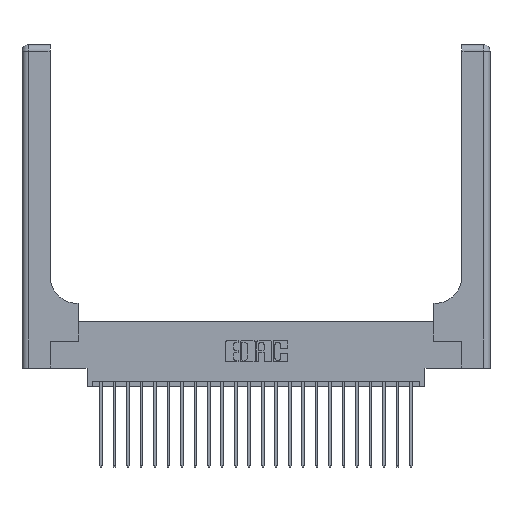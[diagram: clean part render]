
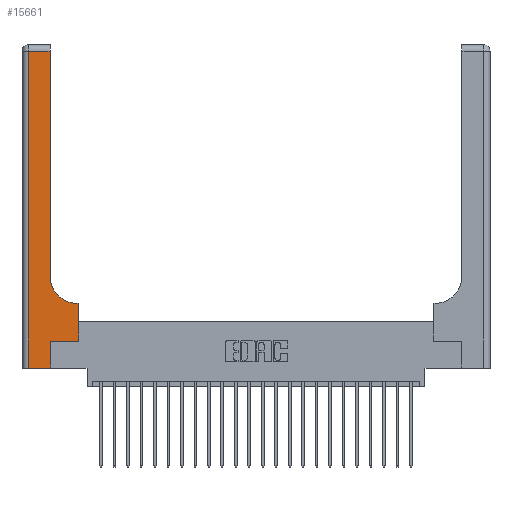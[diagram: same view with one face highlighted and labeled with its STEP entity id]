
A CAD part, top view. The second image highlights one B-rep face of the part: STEP entity #15661.
In plain terms, the highlighted planar face has unit normal (0, 0, 1).
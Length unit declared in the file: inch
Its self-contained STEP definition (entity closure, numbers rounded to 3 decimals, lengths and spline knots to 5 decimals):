
#237 = CARTESIAN_POINT ( 'NONE',  ( 0., 0., 0.37 ) ) ;
#488 = LINE ( 'NONE', #237, #18626 ) ;
#967 = EDGE_CURVE ( 'NONE', #19670, #8756, #488, .T. ) ;
#992 = CARTESIAN_POINT ( 'NONE',  ( 0.06, 2.94, 0.37 ) ) ;
#1204 = DIRECTION ( 'NONE',  ( 0., 1., 0. ) ) ;
#1926 = CARTESIAN_POINT ( 'NONE',  ( 0.26, 0.6, 0.37 ) ) ;
#2576 = FACE_OUTER_BOUND ( 'NONE', #18831, .T. ) ;
#2588 = ORIENTED_EDGE ( 'NONE', *, *, #967, .T. ) ;
#2594 = CARTESIAN_POINT ( 'NONE',  ( 0.528, 0.6, 0.37 ) ) ;
#3532 = VECTOR ( 'NONE', #5127, 39.37008 ) ;
#3684 = LINE ( 'NONE', #22855, #7391 ) ;
#3743 = CIRCLE ( 'NONE', #11062, 0.25 ) ;
#3860 = EDGE_CURVE ( 'NONE', #8756, #13955, #13489, .T. ) ;
#4247 = DIRECTION ( 'NONE',  ( 0., 1., 0. ) ) ;
#4313 = ORIENTED_EDGE ( 'NONE', *, *, #20091, .T. ) ;
#4708 = CARTESIAN_POINT ( 'NONE',  ( 0.51, 0.85, 0.37 ) ) ;
#4880 = ORIENTED_EDGE ( 'NONE', *, *, #19027, .T. ) ;
#5127 = DIRECTION ( 'NONE',  ( 0., -1., 0. ) ) ;
#5379 = EDGE_CURVE ( 'NONE', #11005, #16145, #3743, .T. ) ;
#5455 = ORIENTED_EDGE ( 'NONE', *, *, #5379, .T. ) ;
#5693 = CARTESIAN_POINT ( 'NONE',  ( 0.528, 0.25, 0.37 ) ) ;
#5942 = VECTOR ( 'NONE', #9267, 39.37008 ) ;
#6508 = VERTEX_POINT ( 'NONE', #5693 ) ;
#6538 = DIRECTION ( 'NONE',  ( 1., 0., 0. ) ) ;
#6734 = DIRECTION ( 'NONE',  ( 1., 0., 0. ) ) ;
#7391 = VECTOR ( 'NONE', #1204, 39.37008 ) ;
#7594 = CARTESIAN_POINT ( 'NONE',  ( 0., 2.94, 0.37 ) ) ;
#8018 = ORIENTED_EDGE ( 'NONE', *, *, #3860, .T. ) ;
#8756 = VERTEX_POINT ( 'NONE', #18287 ) ;
#8937 = LINE ( 'NONE', #7594, #17926 ) ;
#9029 = LINE ( 'NONE', #21136, #18025 ) ;
#9267 = DIRECTION ( 'NONE',  ( -1., 0., 0. ) ) ;
#10164 = VECTOR ( 'NONE', #4247, 39.37008 ) ;
#10282 = EDGE_CURVE ( 'NONE', #20040, #19670, #13766, .T. ) ;
#10792 = LINE ( 'NONE', #1926, #5942 ) ;
#10794 = DIRECTION ( 'NONE',  ( 0., 0., -1. ) ) ;
#11005 = VERTEX_POINT ( 'NONE', #16335 ) ;
#11062 = AXIS2_PLACEMENT_3D ( 'NONE', #4708, #17322, #6538 ) ;
#11717 = ORIENTED_EDGE ( 'NONE', *, *, #10282, .T. ) ;
#12171 = CARTESIAN_POINT ( 'NONE',  ( 0.26, 2.94, 0.37 ) ) ;
#12916 = VECTOR ( 'NONE', #20669, 39.37008 ) ;
#13224 = CARTESIAN_POINT ( 'NONE',  ( 0.265, 0.25, 0.37 ) ) ;
#13489 = LINE ( 'NONE', #18871, #12916 ) ;
#13766 = LINE ( 'NONE', #15930, #3532 ) ;
#13876 = EDGE_CURVE ( 'NONE', #18035, #20040, #8937, .T. ) ;
#13947 = ORIENTED_EDGE ( 'NONE', *, *, #20506, .T. ) ;
#13955 = VERTEX_POINT ( 'NONE', #13224 ) ;
#14909 = LINE ( 'NONE', #20425, #10164 ) ;
#15320 = VERTEX_POINT ( 'NONE', #2594 ) ;
#15327 = ORIENTED_EDGE ( 'NONE', *, *, #16107, .T. ) ;
#15661 = ADVANCED_FACE ( 'NONE', ( #2576 ), #21524, .F. ) ;
#15843 = CARTESIAN_POINT ( 'NONE',  ( 0.26, 0.85, 0.37 ) ) ;
#15930 = CARTESIAN_POINT ( 'NONE',  ( 0.06, 3., 0.37 ) ) ;
#16107 = EDGE_CURVE ( 'NONE', #16145, #18035, #3684, .T. ) ;
#16145 = VERTEX_POINT ( 'NONE', #15843 ) ;
#16335 = CARTESIAN_POINT ( 'NONE',  ( 0.51, 0.6, 0.37 ) ) ;
#17322 = DIRECTION ( 'NONE',  ( 0., 0., -1. ) ) ;
#17645 = AXIS2_PLACEMENT_3D ( 'NONE', #17826, #10794, #23332 ) ;
#17826 = CARTESIAN_POINT ( 'NONE',  ( 0., 3., 0.37 ) ) ;
#17926 = VECTOR ( 'NONE', #21996, 39.37008 ) ;
#18025 = VECTOR ( 'NONE', #6734, 39.37008 ) ;
#18035 = VERTEX_POINT ( 'NONE', #12171 ) ;
#18287 = CARTESIAN_POINT ( 'NONE',  ( 0.265, 0., 0.37 ) ) ;
#18380 = DIRECTION ( 'NONE',  ( 1., 0., 0. ) ) ;
#18626 = VECTOR ( 'NONE', #18380, 39.37008 ) ;
#18831 = EDGE_LOOP ( 'NONE', ( #15327, #20113, #11717, #2588, #8018, #4313, #13947, #4880, #5455 ) ) ;
#18871 = CARTESIAN_POINT ( 'NONE',  ( 0.265, 0., 0.37 ) ) ;
#19027 = EDGE_CURVE ( 'NONE', #15320, #11005, #10792, .T. ) ;
#19670 = VERTEX_POINT ( 'NONE', #19833 ) ;
#19833 = CARTESIAN_POINT ( 'NONE',  ( 0.06, 0., 0.37 ) ) ;
#20040 = VERTEX_POINT ( 'NONE', #992 ) ;
#20091 = EDGE_CURVE ( 'NONE', #13955, #6508, #9029, .T. ) ;
#20113 = ORIENTED_EDGE ( 'NONE', *, *, #13876, .T. ) ;
#20425 = CARTESIAN_POINT ( 'NONE',  ( 0.528, 0.25, 0.37 ) ) ;
#20506 = EDGE_CURVE ( 'NONE', #6508, #15320, #14909, .T. ) ;
#20669 = DIRECTION ( 'NONE',  ( 0., 1., 0. ) ) ;
#21136 = CARTESIAN_POINT ( 'NONE',  ( 0.265, 0.25, 0.37 ) ) ;
#21524 = PLANE ( 'NONE',  #17645 ) ;
#21996 = DIRECTION ( 'NONE',  ( -1., 0., 0. ) ) ;
#22855 = CARTESIAN_POINT ( 'NONE',  ( 0.26, 3., 0.37 ) ) ;
#23332 = DIRECTION ( 'NONE',  ( -1., 0., 0. ) ) ;
